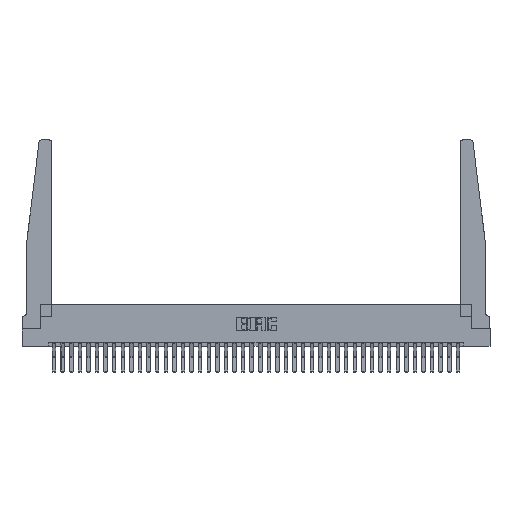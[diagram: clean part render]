
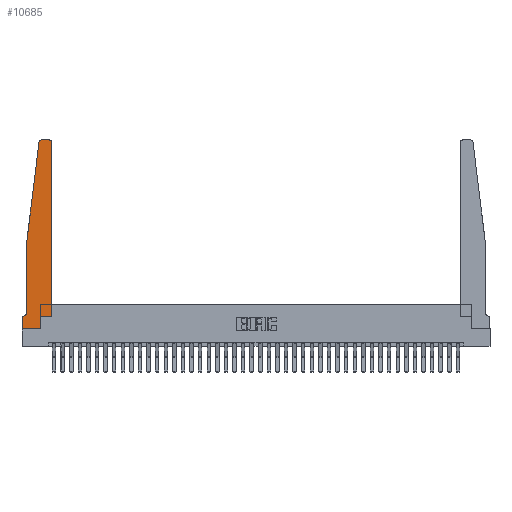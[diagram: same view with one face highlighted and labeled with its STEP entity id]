
A CAD part, top view. The second image highlights one B-rep face of the part: STEP entity #10685.
In plain terms, the highlighted planar face has unit normal (0, 0, 1).
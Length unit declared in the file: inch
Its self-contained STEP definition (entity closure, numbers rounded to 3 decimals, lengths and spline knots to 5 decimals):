
#489 = EDGE_CURVE ( 'NONE', #9078, #19716, #32439, .T. ) ;
#1331 = VECTOR ( 'NONE', #23985, 39.37008 ) ;
#1844 = PLANE ( 'NONE',  #19305 ) ;
#2106 = VERTEX_POINT ( 'NONE', #16474 ) ;
#2170 = ORIENTED_EDGE ( 'NONE', *, *, #32519, .T. ) ;
#2188 = VERTEX_POINT ( 'NONE', #27700 ) ;
#2232 = ORIENTED_EDGE ( 'NONE', *, *, #3631, .T. ) ;
#2566 = CARTESIAN_POINT ( 'NONE',  ( 0., 0., 0.37 ) ) ;
#2612 = DIRECTION ( 'NONE',  ( 1., 0., 0. ) ) ;
#3210 = CARTESIAN_POINT ( 'NONE',  ( 0.2605, 0., 0.37 ) ) ;
#3449 = CARTESIAN_POINT ( 'NONE',  ( 0.015, 0.2375, 0.37 ) ) ;
#3499 = CIRCLE ( 'NONE', #6130, 0.05 ) ;
#3569 = CARTESIAN_POINT ( 'NONE',  ( 0.065, 0.1875, 0.37 ) ) ;
#3631 = EDGE_CURVE ( 'NONE', #9076, #23409, #28759, .T. ) ;
#6130 = AXIS2_PLACEMENT_3D ( 'NONE', #3449, #6342, #28119 ) ;
#6161 = LINE ( 'NONE', #16657, #33104 ) ;
#6184 = ORIENTED_EDGE ( 'NONE', *, *, #32799, .T. ) ;
#6342 = DIRECTION ( 'NONE',  ( 0., 0., -1. ) ) ;
#6904 = ORIENTED_EDGE ( 'NONE', *, *, #12467, .T. ) ;
#7048 = EDGE_LOOP ( 'NONE', ( #31848, #2232, #22468, #21476, #6904, #26330, #9114, #14377, #2170, #20355, #23197, #6184 ) ) ;
#7370 = CARTESIAN_POINT ( 'NONE',  ( 0.395, 2.75, 0.37 ) ) ;
#8224 = LINE ( 'NONE', #21947, #12974 ) ;
#8419 = DIRECTION ( 'NONE',  ( 1., 0., 0. ) ) ;
#8655 = CARTESIAN_POINT ( 'NONE',  ( 0., 0., 0.37 ) ) ;
#9076 = VERTEX_POINT ( 'NONE', #11410 ) ;
#9078 = VERTEX_POINT ( 'NONE', #9135 ) ;
#9114 = ORIENTED_EDGE ( 'NONE', *, *, #489, .T. ) ;
#9135 = CARTESIAN_POINT ( 'NONE',  ( 0., 0.1875, 0.37 ) ) ;
#9755 = EDGE_CURVE ( 'NONE', #26091, #9078, #32818, .T. ) ;
#10240 = CARTESIAN_POINT ( 'NONE',  ( 0.425, 0.18, 0.37 ) ) ;
#10609 = LINE ( 'NONE', #11582, #11014 ) ;
#10685 = ADVANCED_FACE ( 'NONE', ( #15689 ), #1844, .T. ) ;
#11014 = VECTOR ( 'NONE', #30429, 39.37008 ) ;
#11190 = CARTESIAN_POINT ( 'NONE',  ( 0.065, 1.25, 0.37 ) ) ;
#11410 = CARTESIAN_POINT ( 'NONE',  ( 0.27653, 2.75, 0.37 ) ) ;
#11583 = EDGE_CURVE ( 'NONE', #15847, #9076, #6161, .T. ) ;
#11582 = CARTESIAN_POINT ( 'NONE',  ( 0.065, 1.25, 0.37 ) ) ;
#11747 = DIRECTION ( 'NONE',  ( -1., 0., 0. ) ) ;
#12467 = EDGE_CURVE ( 'NONE', #25938, #26091, #3499, .T. ) ;
#12822 = VECTOR ( 'NONE', #16707, 39.37008 ) ;
#12974 = VECTOR ( 'NONE', #8419, 39.37008 ) ;
#13745 = CARTESIAN_POINT ( 'NONE',  ( 0.425, 2.72, 0.37 ) ) ;
#13865 = EDGE_CURVE ( 'NONE', #19716, #18164, #28691, .T. ) ;
#14174 = LINE ( 'NONE', #10240, #1331 ) ;
#14377 = ORIENTED_EDGE ( 'NONE', *, *, #13865, .T. ) ;
#14945 = VECTOR ( 'NONE', #33044, 39.37008 ) ;
#15689 = FACE_OUTER_BOUND ( 'NONE', #7048, .T. ) ;
#15752 = CARTESIAN_POINT ( 'NONE',  ( 0.065, 0.2375, 0.37 ) ) ;
#15847 = VERTEX_POINT ( 'NONE', #7370 ) ;
#16474 = CARTESIAN_POINT ( 'NONE',  ( 0.425, 0.18, 0.37 ) ) ;
#16657 = CARTESIAN_POINT ( 'NONE',  ( 0.25, 2.75, 0.37 ) ) ;
#16707 = DIRECTION ( 'NONE',  ( 0., -1., 0. ) ) ;
#16798 = CARTESIAN_POINT ( 'NONE',  ( 0.395, 2.72, 0.37 ) ) ;
#17254 = CARTESIAN_POINT ( 'NONE',  ( 0.24675, 2.72367, 0.37 ) ) ;
#17801 = EDGE_CURVE ( 'NONE', #19479, #25938, #23938, .T. ) ;
#18164 = VERTEX_POINT ( 'NONE', #3210 ) ;
#19305 = AXIS2_PLACEMENT_3D ( 'NONE', #26490, #34738, #21354 ) ;
#19395 = DIRECTION ( 'NONE',  ( 0., 0., 1. ) ) ;
#19479 = VERTEX_POINT ( 'NONE', #35367 ) ;
#19716 = VERTEX_POINT ( 'NONE', #8655 ) ;
#20355 = ORIENTED_EDGE ( 'NONE', *, *, #26630, .T. ) ;
#20563 = VECTOR ( 'NONE', #21099, 39.37008 ) ;
#21099 = DIRECTION ( 'NONE',  ( 0., 1., 0. ) ) ;
#21354 = DIRECTION ( 'NONE',  ( 1., 0., 0. ) ) ;
#21458 = CARTESIAN_POINT ( 'NONE',  ( 0.2605, 0.18, 0.37 ) ) ;
#21476 = ORIENTED_EDGE ( 'NONE', *, *, #17801, .T. ) ;
#21659 = DIRECTION ( 'NONE',  ( 0., 0., 1. ) ) ;
#21947 = CARTESIAN_POINT ( 'NONE',  ( 0.425, 0.18, 0.37 ) ) ;
#22009 = CARTESIAN_POINT ( 'NONE',  ( 0.27653, 2.72, 0.37 ) ) ;
#22468 = ORIENTED_EDGE ( 'NONE', *, *, #35261, .T. ) ;
#22981 = VECTOR ( 'NONE', #11747, 39.37008 ) ;
#23197 = ORIENTED_EDGE ( 'NONE', *, *, #32589, .T. ) ;
#23409 = VERTEX_POINT ( 'NONE', #17254 ) ;
#23938 = LINE ( 'NONE', #11190, #14945 ) ;
#23985 = DIRECTION ( 'NONE',  ( 0., 1., 0. ) ) ;
#25938 = VERTEX_POINT ( 'NONE', #15752 ) ;
#26091 = VERTEX_POINT ( 'NONE', #27235 ) ;
#26330 = ORIENTED_EDGE ( 'NONE', *, *, #9755, .T. ) ;
#26490 = CARTESIAN_POINT ( 'NONE',  ( 0., 0.1875, 0.37 ) ) ;
#26630 = EDGE_CURVE ( 'NONE', #2188, #2106, #8224, .T. ) ;
#27163 = VERTEX_POINT ( 'NONE', #13745 ) ;
#27235 = CARTESIAN_POINT ( 'NONE',  ( 0.015, 0.1875, 0.37 ) ) ;
#27700 = CARTESIAN_POINT ( 'NONE',  ( 0.2605, 0.18, 0.37 ) ) ;
#28119 = DIRECTION ( 'NONE',  ( -1., 0., 0. ) ) ;
#28691 = LINE ( 'NONE', #2566, #34220 ) ;
#28759 = CIRCLE ( 'NONE', #32609, 0.03 ) ;
#28838 = AXIS2_PLACEMENT_3D ( 'NONE', #16798, #19395, #30263 ) ;
#29968 = CIRCLE ( 'NONE', #28838, 0.03 ) ;
#30263 = DIRECTION ( 'NONE',  ( 1., 0., 0. ) ) ;
#30429 = DIRECTION ( 'NONE',  ( -0.122, -0.992, 0. ) ) ;
#30484 = DIRECTION ( 'NONE',  ( -1., 0., 0. ) ) ;
#31848 = ORIENTED_EDGE ( 'NONE', *, *, #11583, .T. ) ;
#32439 = LINE ( 'NONE', #33051, #12822 ) ;
#32519 = EDGE_CURVE ( 'NONE', #18164, #2188, #35103, .T. ) ;
#32589 = EDGE_CURVE ( 'NONE', #2106, #27163, #14174, .T. ) ;
#32609 = AXIS2_PLACEMENT_3D ( 'NONE', #22009, #21659, #2612 ) ;
#32799 = EDGE_CURVE ( 'NONE', #27163, #15847, #29968, .T. ) ;
#32818 = LINE ( 'NONE', #3569, #22981 ) ;
#33044 = DIRECTION ( 'NONE',  ( 0., -1., 0. ) ) ;
#33051 = CARTESIAN_POINT ( 'NONE',  ( 0., 0., 0.37 ) ) ;
#33104 = VECTOR ( 'NONE', #30484, 39.37008 ) ;
#34145 = DIRECTION ( 'NONE',  ( 1., 0., 0. ) ) ;
#34220 = VECTOR ( 'NONE', #34145, 39.37008 ) ;
#34738 = DIRECTION ( 'NONE',  ( 0., 0., 1. ) ) ;
#35103 = LINE ( 'NONE', #21458, #20563 ) ;
#35261 = EDGE_CURVE ( 'NONE', #23409, #19479, #10609, .T. ) ;
#35367 = CARTESIAN_POINT ( 'NONE',  ( 0.065, 1.25, 0.37 ) ) ;
